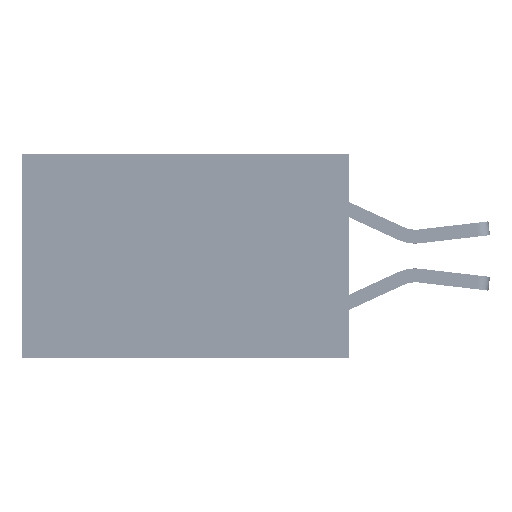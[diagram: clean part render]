
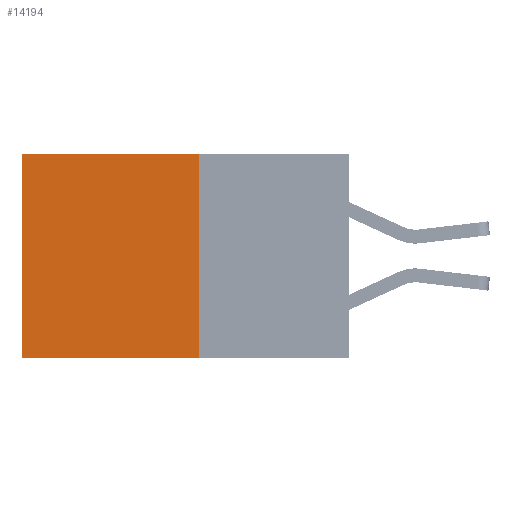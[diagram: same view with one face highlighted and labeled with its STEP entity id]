
A CAD part, left-side view. The second image highlights one B-rep face of the part: STEP entity #14194.
In plain terms, the highlighted planar face has unit normal (-1, 0, 0).
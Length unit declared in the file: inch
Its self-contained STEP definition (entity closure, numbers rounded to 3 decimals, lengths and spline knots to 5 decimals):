
#74 = CARTESIAN_POINT ( 'NONE',  ( 0.277, 0.27, 0. ) ) ;
#432 = CARTESIAN_POINT ( 'NONE',  ( 0.277, 0.27, -0.37 ) ) ;
#1221 = ORIENTED_EDGE ( 'NONE', *, *, #21137, .F. ) ;
#1690 = VERTEX_POINT ( 'NONE', #19177 ) ;
#3052 = ORIENTED_EDGE ( 'NONE', *, *, #27962, .F. ) ;
#3055 = LINE ( 'NONE', #25361, #15661 ) ;
#4093 = CARTESIAN_POINT ( 'NONE',  ( 0.277, 0.27, -0.37 ) ) ;
#6222 = EDGE_LOOP ( 'NONE', ( #14972, #3052, #1221, #26223 ) ) ;
#7198 = DIRECTION ( 'NONE',  ( 0., 0., -1. ) ) ;
#7427 = LINE ( 'NONE', #16615, #27123 ) ;
#9542 = VECTOR ( 'NONE', #15071, 39.37008 ) ;
#10151 = FACE_OUTER_BOUND ( 'NONE', #6222, .T. ) ;
#10532 = DIRECTION ( 'NONE',  ( 0., 0., -1. ) ) ;
#12308 = VERTEX_POINT ( 'NONE', #4093 ) ;
#12640 = VERTEX_POINT ( 'NONE', #74 ) ;
#14194 = ADVANCED_FACE ( 'NONE', ( #10151 ), #19620, .F. ) ;
#14464 = EDGE_CURVE ( 'NONE', #25930, #1690, #3055, .T. ) ;
#14626 = CARTESIAN_POINT ( 'NONE',  ( 0.277, 0.27, -0.37 ) ) ;
#14972 = ORIENTED_EDGE ( 'NONE', *, *, #14464, .T. ) ;
#15071 = DIRECTION ( 'NONE',  ( 0., 1., 0. ) ) ;
#15661 = VECTOR ( 'NONE', #10532, 39.37008 ) ;
#16140 = CARTESIAN_POINT ( 'NONE',  ( 0.277, 0.59, 0. ) ) ;
#16615 = CARTESIAN_POINT ( 'NONE',  ( 0.277, 0.27, -0.37 ) ) ;
#17665 = EDGE_CURVE ( 'NONE', #12640, #25930, #23490, .T. ) ;
#18041 = DIRECTION ( 'NONE',  ( 0., 0., -1. ) ) ;
#19177 = CARTESIAN_POINT ( 'NONE',  ( 0.277, 0.59, -0.37 ) ) ;
#19620 = PLANE ( 'NONE',  #26125 ) ;
#21137 = EDGE_CURVE ( 'NONE', #12640, #12308, #31863, .T. ) ;
#22058 = DIRECTION ( 'NONE',  ( 1., 0., 0. ) ) ;
#23490 = LINE ( 'NONE', #27261, #9542 ) ;
#25361 = CARTESIAN_POINT ( 'NONE',  ( 0.277, 0.59, -0.37 ) ) ;
#25930 = VERTEX_POINT ( 'NONE', #16140 ) ;
#26125 = AXIS2_PLACEMENT_3D ( 'NONE', #14626, #22058, #7198 ) ;
#26223 = ORIENTED_EDGE ( 'NONE', *, *, #17665, .T. ) ;
#27123 = VECTOR ( 'NONE', #31132, 39.37008 ) ;
#27261 = CARTESIAN_POINT ( 'NONE',  ( 0.277, 0.27, 0. ) ) ;
#27962 = EDGE_CURVE ( 'NONE', #12308, #1690, #7427, .T. ) ;
#31091 = VECTOR ( 'NONE', #18041, 39.37008 ) ;
#31132 = DIRECTION ( 'NONE',  ( 0., 1., 0. ) ) ;
#31863 = LINE ( 'NONE', #432, #31091 ) ;
